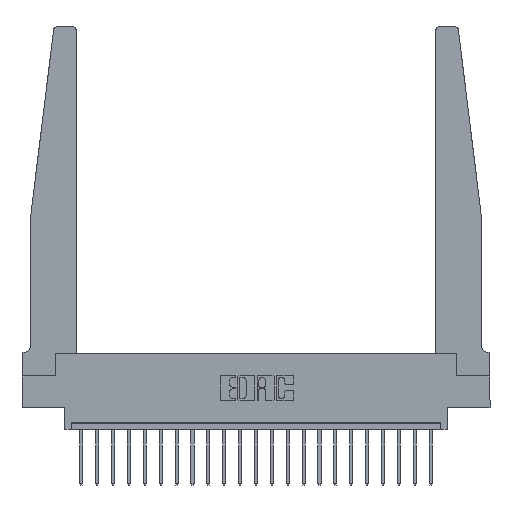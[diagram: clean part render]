
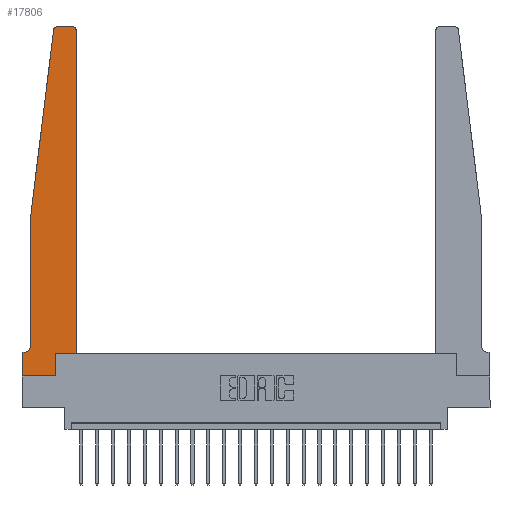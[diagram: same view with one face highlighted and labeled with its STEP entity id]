
A CAD part, top view. The second image highlights one B-rep face of the part: STEP entity #17806.
In plain terms, the highlighted planar face has unit normal (0, 0, 1).
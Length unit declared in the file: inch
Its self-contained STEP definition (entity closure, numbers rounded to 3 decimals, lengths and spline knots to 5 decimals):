
#159 = CARTESIAN_POINT ( 'NONE',  ( 0.2605, 0.18, 0.37 ) ) ;
#492 = CARTESIAN_POINT ( 'NONE',  ( 0.2605, 0.18, 0.37 ) ) ;
#565 = CARTESIAN_POINT ( 'NONE',  ( 0.425, 0.18, 0.37 ) ) ;
#1139 = VECTOR ( 'NONE', #3834, 39.37008 ) ;
#1621 = AXIS2_PLACEMENT_3D ( 'NONE', #16255, #13455, #16629 ) ;
#2020 = CARTESIAN_POINT ( 'NONE',  ( 0.425, 2.72, 0.37 ) ) ;
#2026 = DIRECTION ( 'NONE',  ( 1., 0., 0. ) ) ;
#2027 = DIRECTION ( 'NONE',  ( 0., 0., 1. ) ) ;
#2101 = CARTESIAN_POINT ( 'NONE',  ( 0., 0., 0.37 ) ) ;
#2235 = EDGE_CURVE ( 'NONE', #17403, #20415, #7872, .T. ) ;
#2573 = ORIENTED_EDGE ( 'NONE', *, *, #9744, .T. ) ;
#2683 = VECTOR ( 'NONE', #13500, 39.37008 ) ;
#2870 = CARTESIAN_POINT ( 'NONE',  ( 0.065, 1.25, 0.37 ) ) ;
#3294 = CARTESIAN_POINT ( 'NONE',  ( 0.065, 0.1875, 0.37 ) ) ;
#3447 = LINE ( 'NONE', #2870, #15776 ) ;
#3625 = VECTOR ( 'NONE', #14049, 39.37008 ) ;
#3834 = DIRECTION ( 'NONE',  ( 0., -1., 0. ) ) ;
#4662 = VECTOR ( 'NONE', #7958, 39.37008 ) ;
#4746 = CARTESIAN_POINT ( 'NONE',  ( 0.425, 0.18, 0.37 ) ) ;
#4809 = VERTEX_POINT ( 'NONE', #17634 ) ;
#5231 = DIRECTION ( 'NONE',  ( 0., 0., -1. ) ) ;
#5867 = CIRCLE ( 'NONE', #10722, 0.03 ) ;
#6151 = ORIENTED_EDGE ( 'NONE', *, *, #2235, .T. ) ;
#6153 = ORIENTED_EDGE ( 'NONE', *, *, #17074, .T. ) ;
#6587 = CARTESIAN_POINT ( 'NONE',  ( 0.27653, 2.75, 0.37 ) ) ;
#6629 = VERTEX_POINT ( 'NONE', #6587 ) ;
#7058 = CIRCLE ( 'NONE', #8139, 0.03 ) ;
#7646 = LINE ( 'NONE', #159, #2683 ) ;
#7747 = DIRECTION ( 'NONE',  ( 0., -1., 0. ) ) ;
#7872 = CIRCLE ( 'NONE', #20471, 0.05 ) ;
#7958 = DIRECTION ( 'NONE',  ( 1., 0., 0. ) ) ;
#7966 = ORIENTED_EDGE ( 'NONE', *, *, #17296, .T. ) ;
#8139 = AXIS2_PLACEMENT_3D ( 'NONE', #17781, #11061, #21109 ) ;
#8185 = LINE ( 'NONE', #17676, #15827 ) ;
#8406 = DIRECTION ( 'NONE',  ( -1., 0., 0. ) ) ;
#8440 = ORIENTED_EDGE ( 'NONE', *, *, #18838, .T. ) ;
#8571 = EDGE_LOOP ( 'NONE', ( #12992, #15793, #19408, #8440, #6151, #11663, #7966, #13426, #12369, #2573, #17274, #6153 ) ) ;
#8689 = CARTESIAN_POINT ( 'NONE',  ( 0.065, 0.2375, 0.37 ) ) ;
#8998 = VERTEX_POINT ( 'NONE', #492 ) ;
#9406 = LINE ( 'NONE', #20468, #10469 ) ;
#9744 = EDGE_CURVE ( 'NONE', #8998, #21738, #16253, .T. ) ;
#10051 = LINE ( 'NONE', #3294, #18495 ) ;
#10294 = DIRECTION ( 'NONE',  ( 1., 0., 0. ) ) ;
#10469 = VECTOR ( 'NONE', #2026, 39.37008 ) ;
#10722 = AXIS2_PLACEMENT_3D ( 'NONE', #11969, #2027, #10294 ) ;
#11061 = DIRECTION ( 'NONE',  ( 0., 0., 1. ) ) ;
#11098 = LINE ( 'NONE', #2101, #1139 ) ;
#11663 = ORIENTED_EDGE ( 'NONE', *, *, #12739, .T. ) ;
#11758 = VECTOR ( 'NONE', #13769, 39.37008 ) ;
#11969 = CARTESIAN_POINT ( 'NONE',  ( 0.395, 2.72, 0.37 ) ) ;
#12205 = CARTESIAN_POINT ( 'NONE',  ( 0.065, 1.25, 0.37 ) ) ;
#12369 = ORIENTED_EDGE ( 'NONE', *, *, #18440, .T. ) ;
#12648 = VERTEX_POINT ( 'NONE', #15244 ) ;
#12739 = EDGE_CURVE ( 'NONE', #20415, #18478, #10051, .T. ) ;
#12992 = ORIENTED_EDGE ( 'NONE', *, *, #13175, .T. ) ;
#13175 = EDGE_CURVE ( 'NONE', #12648, #6629, #8185, .T. ) ;
#13426 = ORIENTED_EDGE ( 'NONE', *, *, #19857, .T. ) ;
#13455 = DIRECTION ( 'NONE',  ( 0., 0., 1. ) ) ;
#13500 = DIRECTION ( 'NONE',  ( 0., 1., 0. ) ) ;
#13769 = DIRECTION ( 'NONE',  ( -0.122, -0.992, 0. ) ) ;
#13908 = CARTESIAN_POINT ( 'NONE',  ( 0.065, 1.25, 0.37 ) ) ;
#14049 = DIRECTION ( 'NONE',  ( 0., 1., 0. ) ) ;
#14508 = VERTEX_POINT ( 'NONE', #2020 ) ;
#14560 = PLANE ( 'NONE',  #1621 ) ;
#15244 = CARTESIAN_POINT ( 'NONE',  ( 0.395, 2.75, 0.37 ) ) ;
#15776 = VECTOR ( 'NONE', #7747, 39.37008 ) ;
#15793 = ORIENTED_EDGE ( 'NONE', *, *, #20375, .T. ) ;
#15824 = VERTEX_POINT ( 'NONE', #16323 ) ;
#15827 = VECTOR ( 'NONE', #19360, 39.37008 ) ;
#16248 = LINE ( 'NONE', #565, #3625 ) ;
#16253 = LINE ( 'NONE', #4746, #4662 ) ;
#16255 = CARTESIAN_POINT ( 'NONE',  ( 0., 0.1875, 0.37 ) ) ;
#16323 = CARTESIAN_POINT ( 'NONE',  ( 0.24675, 2.72367, 0.37 ) ) ;
#16629 = DIRECTION ( 'NONE',  ( 1., 0., 0. ) ) ;
#16885 = FACE_OUTER_BOUND ( 'NONE', #8571, .T. ) ;
#16980 = DIRECTION ( 'NONE',  ( -1., 0., 0. ) ) ;
#17074 = EDGE_CURVE ( 'NONE', #14508, #12648, #5867, .T. ) ;
#17274 = ORIENTED_EDGE ( 'NONE', *, *, #21187, .T. ) ;
#17296 = EDGE_CURVE ( 'NONE', #18478, #21129, #11098, .T. ) ;
#17403 = VERTEX_POINT ( 'NONE', #8689 ) ;
#17634 = CARTESIAN_POINT ( 'NONE',  ( 0.2605, 0., 0.37 ) ) ;
#17676 = CARTESIAN_POINT ( 'NONE',  ( 0.25, 2.75, 0.37 ) ) ;
#17781 = CARTESIAN_POINT ( 'NONE',  ( 0.27653, 2.72, 0.37 ) ) ;
#17806 = ADVANCED_FACE ( 'NONE', ( #16885 ), #14560, .T. ) ;
#18092 = LINE ( 'NONE', #12205, #11758 ) ;
#18440 = EDGE_CURVE ( 'NONE', #4809, #8998, #7646, .T. ) ;
#18478 = VERTEX_POINT ( 'NONE', #20073 ) ;
#18495 = VECTOR ( 'NONE', #8406, 39.37008 ) ;
#18838 = EDGE_CURVE ( 'NONE', #21262, #17403, #3447, .T. ) ;
#19360 = DIRECTION ( 'NONE',  ( -1., 0., 0. ) ) ;
#19408 = ORIENTED_EDGE ( 'NONE', *, *, #21240, .T. ) ;
#19667 = CARTESIAN_POINT ( 'NONE',  ( 0., 0., 0.37 ) ) ;
#19857 = EDGE_CURVE ( 'NONE', #21129, #4809, #9406, .T. ) ;
#20054 = CARTESIAN_POINT ( 'NONE',  ( 0.015, 0.1875, 0.37 ) ) ;
#20073 = CARTESIAN_POINT ( 'NONE',  ( 0., 0.1875, 0.37 ) ) ;
#20375 = EDGE_CURVE ( 'NONE', #6629, #15824, #7058, .T. ) ;
#20382 = CARTESIAN_POINT ( 'NONE',  ( 0.015, 0.2375, 0.37 ) ) ;
#20415 = VERTEX_POINT ( 'NONE', #20054 ) ;
#20468 = CARTESIAN_POINT ( 'NONE',  ( 0., 0., 0.37 ) ) ;
#20471 = AXIS2_PLACEMENT_3D ( 'NONE', #20382, #5231, #16980 ) ;
#20674 = CARTESIAN_POINT ( 'NONE',  ( 0.425, 0.18, 0.37 ) ) ;
#21109 = DIRECTION ( 'NONE',  ( 1., 0., 0. ) ) ;
#21129 = VERTEX_POINT ( 'NONE', #19667 ) ;
#21187 = EDGE_CURVE ( 'NONE', #21738, #14508, #16248, .T. ) ;
#21240 = EDGE_CURVE ( 'NONE', #15824, #21262, #18092, .T. ) ;
#21262 = VERTEX_POINT ( 'NONE', #13908 ) ;
#21738 = VERTEX_POINT ( 'NONE', #20674 ) ;
